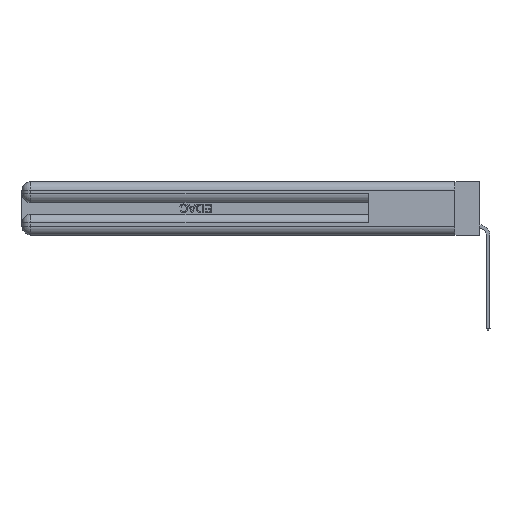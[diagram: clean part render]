
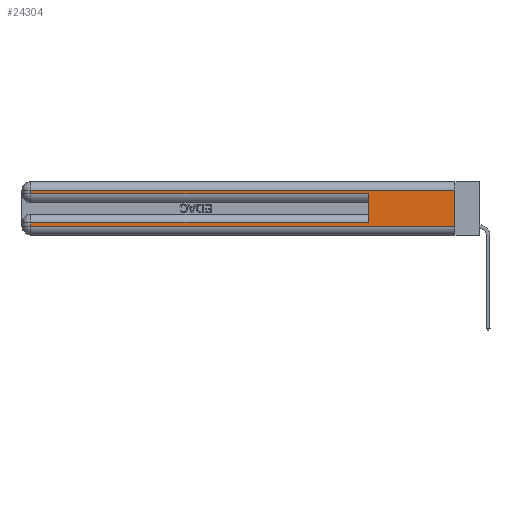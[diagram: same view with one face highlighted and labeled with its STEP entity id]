
A CAD part, left-side view. The second image highlights one B-rep face of the part: STEP entity #24304.
In plain terms, the highlighted planar face has unit normal (-1, 0, 0).
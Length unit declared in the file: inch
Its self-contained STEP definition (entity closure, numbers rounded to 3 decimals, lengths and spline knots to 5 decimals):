
#326 = DIRECTION ( 'NONE',  ( 0., 0., 1. ) ) ;
#1335 = CARTESIAN_POINT ( 'NONE',  ( 0., 0., 0.31 ) ) ;
#2806 = VECTOR ( 'NONE', #34489, 39.37008 ) ;
#3735 = CARTESIAN_POINT ( 'NONE',  ( 0., 2.94, 0.06 ) ) ;
#4084 = PLANE ( 'NONE',  #30102 ) ;
#4311 = CARTESIAN_POINT ( 'NONE',  ( 0., 0., 0.06 ) ) ;
#5155 = DIRECTION ( 'NONE',  ( 0., 0., -1. ) ) ;
#5241 = VECTOR ( 'NONE', #326, 39.37008 ) ;
#6382 = CARTESIAN_POINT ( 'NONE',  ( 0., 2.94, 0.285 ) ) ;
#6409 = CARTESIAN_POINT ( 'NONE',  ( 0., 2.94, 0.31 ) ) ;
#6510 = CARTESIAN_POINT ( 'NONE',  ( 0., 0.6, 0.285 ) ) ;
#9354 = EDGE_CURVE ( 'NONE', #29423, #27538, #17373, .T. ) ;
#9600 = CARTESIAN_POINT ( 'NONE',  ( 0., 0., 0.085 ) ) ;
#9681 = DIRECTION ( 'NONE',  ( 0., 0., -1. ) ) ;
#9814 = EDGE_CURVE ( 'NONE', #29846, #18933, #10151, .T. ) ;
#9980 = ORIENTED_EDGE ( 'NONE', *, *, #29965, .T. ) ;
#10151 = LINE ( 'NONE', #30732, #24519 ) ;
#10180 = CARTESIAN_POINT ( 'NONE',  ( 0., 0., 0.06 ) ) ;
#10231 = VERTEX_POINT ( 'NONE', #35256 ) ;
#10299 = CARTESIAN_POINT ( 'NONE',  ( 0., 0.6, 0.085 ) ) ;
#10905 = ORIENTED_EDGE ( 'NONE', *, *, #27373, .F. ) ;
#12166 = LINE ( 'NONE', #16049, #20193 ) ;
#12711 = VECTOR ( 'NONE', #25793, 39.37008 ) ;
#13538 = LINE ( 'NONE', #9600, #12711 ) ;
#13639 = FACE_OUTER_BOUND ( 'NONE', #27691, .T. ) ;
#13940 = VERTEX_POINT ( 'NONE', #6510 ) ;
#14543 = DIRECTION ( 'NONE',  ( 0., 0., -1. ) ) ;
#16049 = CARTESIAN_POINT ( 'NONE',  ( 0., 0., 0.37 ) ) ;
#17079 = LINE ( 'NONE', #4311, #30617 ) ;
#17373 = LINE ( 'NONE', #18239, #2806 ) ;
#17426 = DIRECTION ( 'NONE',  ( 0., -1., 0. ) ) ;
#17808 = ORIENTED_EDGE ( 'NONE', *, *, #9814, .T. ) ;
#18183 = CARTESIAN_POINT ( 'NONE',  ( 0., 2.94, 0.085 ) ) ;
#18239 = CARTESIAN_POINT ( 'NONE',  ( 0., 2.94, 0.37 ) ) ;
#18518 = VECTOR ( 'NONE', #23308, 39.37008 ) ;
#18933 = VERTEX_POINT ( 'NONE', #6382 ) ;
#19535 = ORIENTED_EDGE ( 'NONE', *, *, #22449, .T. ) ;
#20193 = VECTOR ( 'NONE', #5155, 39.37008 ) ;
#21572 = VECTOR ( 'NONE', #17426, 39.37008 ) ;
#22099 = ORIENTED_EDGE ( 'NONE', *, *, #32293, .T. ) ;
#22310 = ORIENTED_EDGE ( 'NONE', *, *, #27835, .F. ) ;
#22449 = EDGE_CURVE ( 'NONE', #10231, #29846, #25721, .T. ) ;
#22540 = VERTEX_POINT ( 'NONE', #10180 ) ;
#23150 = CARTESIAN_POINT ( 'NONE',  ( 0., 0., 0.37 ) ) ;
#23308 = DIRECTION ( 'NONE',  ( 0., 1., 0. ) ) ;
#24304 = ADVANCED_FACE ( 'NONE', ( #13639 ), #4084, .F. ) ;
#24519 = VECTOR ( 'NONE', #14543, 39.37008 ) ;
#25604 = EDGE_CURVE ( 'NONE', #32525, #29423, #13538, .T. ) ;
#25721 = LINE ( 'NONE', #1335, #18518 ) ;
#25793 = DIRECTION ( 'NONE',  ( 0., 1., 0. ) ) ;
#25885 = DIRECTION ( 'NONE',  ( 1., 0., 0. ) ) ;
#26097 = DIRECTION ( 'NONE',  ( 0., -1., 0. ) ) ;
#27373 = EDGE_CURVE ( 'NONE', #32525, #13940, #34178, .T. ) ;
#27538 = VERTEX_POINT ( 'NONE', #3735 ) ;
#27691 = EDGE_LOOP ( 'NONE', ( #22310, #19535, #17808, #22099, #10905, #34580, #28617, #9980 ) ) ;
#27835 = EDGE_CURVE ( 'NONE', #10231, #22540, #12166, .T. ) ;
#28617 = ORIENTED_EDGE ( 'NONE', *, *, #9354, .T. ) ;
#28782 = LINE ( 'NONE', #30908, #21572 ) ;
#29423 = VERTEX_POINT ( 'NONE', #18183 ) ;
#29846 = VERTEX_POINT ( 'NONE', #6409 ) ;
#29965 = EDGE_CURVE ( 'NONE', #27538, #22540, #17079, .T. ) ;
#30102 = AXIS2_PLACEMENT_3D ( 'NONE', #23150, #25885, #9681 ) ;
#30617 = VECTOR ( 'NONE', #26097, 39.37008 ) ;
#30732 = CARTESIAN_POINT ( 'NONE',  ( 0., 2.94, 0.37 ) ) ;
#30908 = CARTESIAN_POINT ( 'NONE',  ( 0., 0., 0.285 ) ) ;
#32293 = EDGE_CURVE ( 'NONE', #18933, #13940, #28782, .T. ) ;
#32525 = VERTEX_POINT ( 'NONE', #10299 ) ;
#32997 = CARTESIAN_POINT ( 'NONE',  ( 0., 0.6, 0.145 ) ) ;
#34178 = LINE ( 'NONE', #32997, #5241 ) ;
#34489 = DIRECTION ( 'NONE',  ( 0., 0., -1. ) ) ;
#34580 = ORIENTED_EDGE ( 'NONE', *, *, #25604, .T. ) ;
#35256 = CARTESIAN_POINT ( 'NONE',  ( 0., 0., 0.31 ) ) ;
